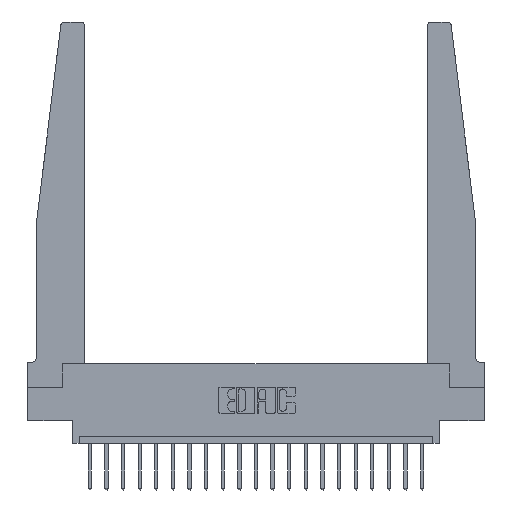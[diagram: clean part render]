
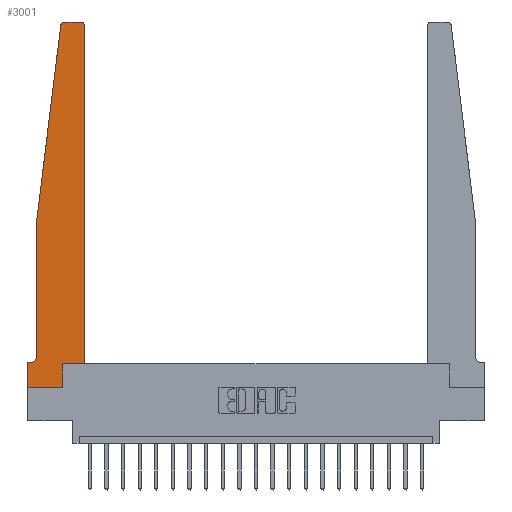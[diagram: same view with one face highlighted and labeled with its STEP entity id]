
A CAD part, top view. The second image highlights one B-rep face of the part: STEP entity #3001.
In plain terms, the highlighted planar face has unit normal (0, 0, 1).
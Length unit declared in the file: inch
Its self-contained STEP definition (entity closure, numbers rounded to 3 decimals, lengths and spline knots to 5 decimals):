
#333 = CARTESIAN_POINT ( 'NONE',  ( 0.015, 0.1875, 0.37 ) ) ;
#1010 = VECTOR ( 'NONE', #8053, 39.37008 ) ;
#1022 = PLANE ( 'NONE',  #12122 ) ;
#1224 = CARTESIAN_POINT ( 'NONE',  ( 0., 0.1875, 0.37 ) ) ;
#1341 = VERTEX_POINT ( 'NONE', #3713 ) ;
#1450 = VECTOR ( 'NONE', #2844, 39.37008 ) ;
#1490 = VERTEX_POINT ( 'NONE', #19080 ) ;
#1991 = CARTESIAN_POINT ( 'NONE',  ( 0.24675, 2.72367, 0.37 ) ) ;
#2009 = LINE ( 'NONE', #3826, #7385 ) ;
#2108 = ORIENTED_EDGE ( 'NONE', *, *, #13648, .T. ) ;
#2255 = CARTESIAN_POINT ( 'NONE',  ( 0.065, 0.2375, 0.37 ) ) ;
#2844 = DIRECTION ( 'NONE',  ( 0., -1., 0. ) ) ;
#3001 = ADVANCED_FACE ( 'NONE', ( #9588 ), #1022, .T. ) ;
#3008 = CARTESIAN_POINT ( 'NONE',  ( 0., 0.1875, 0.37 ) ) ;
#3049 = CARTESIAN_POINT ( 'NONE',  ( 0.065, 0.1875, 0.37 ) ) ;
#3063 = LINE ( 'NONE', #8006, #19202 ) ;
#3083 = ORIENTED_EDGE ( 'NONE', *, *, #13644, .T. ) ;
#3428 = CARTESIAN_POINT ( 'NONE',  ( 0.2605, 0.18, 0.37 ) ) ;
#3634 = ORIENTED_EDGE ( 'NONE', *, *, #11087, .T. ) ;
#3713 = CARTESIAN_POINT ( 'NONE',  ( 0.425, 2.72, 0.37 ) ) ;
#3826 = CARTESIAN_POINT ( 'NONE',  ( 0., 0., 0.37 ) ) ;
#4014 = VECTOR ( 'NONE', #17731, 39.37008 ) ;
#4241 = CARTESIAN_POINT ( 'NONE',  ( 0.27653, 2.75, 0.37 ) ) ;
#5000 = VECTOR ( 'NONE', #10655, 39.37008 ) ;
#5404 = CARTESIAN_POINT ( 'NONE',  ( 0., 0., 0.37 ) ) ;
#5937 = VERTEX_POINT ( 'NONE', #4241 ) ;
#5967 = DIRECTION ( 'NONE',  ( 0., 0., -1. ) ) ;
#6072 = CARTESIAN_POINT ( 'NONE',  ( 0., 0., 0.37 ) ) ;
#6158 = LINE ( 'NONE', #12679, #13641 ) ;
#6298 = VERTEX_POINT ( 'NONE', #3008 ) ;
#7385 = VECTOR ( 'NONE', #16719, 39.37008 ) ;
#7458 = AXIS2_PLACEMENT_3D ( 'NONE', #17946, #7973, #19352 ) ;
#7587 = VERTEX_POINT ( 'NONE', #2255 ) ;
#7666 = ORIENTED_EDGE ( 'NONE', *, *, #9296, .T. ) ;
#7973 = DIRECTION ( 'NONE',  ( 0., 0., 1. ) ) ;
#8006 = CARTESIAN_POINT ( 'NONE',  ( 0.065, 1.25, 0.37 ) ) ;
#8022 = ORIENTED_EDGE ( 'NONE', *, *, #17129, .T. ) ;
#8035 = CARTESIAN_POINT ( 'NONE',  ( 0.2605, 0., 0.37 ) ) ;
#8053 = DIRECTION ( 'NONE',  ( 0., 1., 0. ) ) ;
#8662 = EDGE_CURVE ( 'NONE', #17371, #16369, #2009, .T. ) ;
#9296 = EDGE_CURVE ( 'NONE', #13690, #5937, #17333, .T. ) ;
#9581 = DIRECTION ( 'NONE',  ( 1., 0., 0. ) ) ;
#9588 = FACE_OUTER_BOUND ( 'NONE', #10808, .T. ) ;
#9617 = CARTESIAN_POINT ( 'NONE',  ( 0.27653, 2.72, 0.37 ) ) ;
#9764 = ORIENTED_EDGE ( 'NONE', *, *, #12381, .T. ) ;
#10095 = VERTEX_POINT ( 'NONE', #15756 ) ;
#10655 = DIRECTION ( 'NONE',  ( -1., 0., 0. ) ) ;
#10656 = CARTESIAN_POINT ( 'NONE',  ( 0.015, 0.2375, 0.37 ) ) ;
#10808 = EDGE_LOOP ( 'NONE', ( #7666, #12319, #2108, #3634, #8022, #19317, #12587, #10823, #12771, #9764, #3083, #17591 ) ) ;
#10823 = ORIENTED_EDGE ( 'NONE', *, *, #8662, .T. ) ;
#11057 = EDGE_CURVE ( 'NONE', #1341, #13690, #15687, .T. ) ;
#11087 = EDGE_CURVE ( 'NONE', #18530, #7587, #14510, .T. ) ;
#11091 = CARTESIAN_POINT ( 'NONE',  ( 0.425, 0.18, 0.37 ) ) ;
#11159 = CARTESIAN_POINT ( 'NONE',  ( 0.065, 1.25, 0.37 ) ) ;
#11291 = VERTEX_POINT ( 'NONE', #333 ) ;
#11306 = LINE ( 'NONE', #11091, #15420 ) ;
#11911 = DIRECTION ( 'NONE',  ( 1., 0., 0. ) ) ;
#12122 = AXIS2_PLACEMENT_3D ( 'NONE', #1224, #15833, #17431 ) ;
#12319 = ORIENTED_EDGE ( 'NONE', *, *, #15755, .T. ) ;
#12381 = EDGE_CURVE ( 'NONE', #1490, #10095, #6158, .T. ) ;
#12587 = ORIENTED_EDGE ( 'NONE', *, *, #17140, .T. ) ;
#12679 = CARTESIAN_POINT ( 'NONE',  ( 0.425, 0.18, 0.37 ) ) ;
#12771 = ORIENTED_EDGE ( 'NONE', *, *, #12784, .T. ) ;
#12784 = EDGE_CURVE ( 'NONE', #16369, #1490, #19767, .T. ) ;
#13641 = VECTOR ( 'NONE', #9581, 39.37008 ) ;
#13644 = EDGE_CURVE ( 'NONE', #10095, #1341, #11306, .T. ) ;
#13648 = EDGE_CURVE ( 'NONE', #20662, #18530, #3063, .T. ) ;
#13690 = VERTEX_POINT ( 'NONE', #16057 ) ;
#14204 = DIRECTION ( 'NONE',  ( -1., 0., 0. ) ) ;
#14510 = LINE ( 'NONE', #11159, #4014 ) ;
#14543 = DIRECTION ( 'NONE',  ( -0.122, -0.992, 0. ) ) ;
#14750 = DIRECTION ( 'NONE',  ( 0., 1., 0. ) ) ;
#14859 = VECTOR ( 'NONE', #17550, 39.37008 ) ;
#15151 = DIRECTION ( 'NONE',  ( 0., 0., 1. ) ) ;
#15420 = VECTOR ( 'NONE', #14750, 39.37008 ) ;
#15502 = CIRCLE ( 'NONE', #18238, 0.05 ) ;
#15687 = CIRCLE ( 'NONE', #7458, 0.03 ) ;
#15755 = EDGE_CURVE ( 'NONE', #5937, #20662, #17175, .T. ) ;
#15756 = CARTESIAN_POINT ( 'NONE',  ( 0.425, 0.18, 0.37 ) ) ;
#15800 = AXIS2_PLACEMENT_3D ( 'NONE', #9617, #15151, #11911 ) ;
#15833 = DIRECTION ( 'NONE',  ( 0., 0., 1. ) ) ;
#16057 = CARTESIAN_POINT ( 'NONE',  ( 0.395, 2.75, 0.37 ) ) ;
#16156 = LINE ( 'NONE', #3049, #14859 ) ;
#16369 = VERTEX_POINT ( 'NONE', #8035 ) ;
#16719 = DIRECTION ( 'NONE',  ( 1., 0., 0. ) ) ;
#17129 = EDGE_CURVE ( 'NONE', #7587, #11291, #15502, .T. ) ;
#17140 = EDGE_CURVE ( 'NONE', #6298, #17371, #20773, .T. ) ;
#17175 = CIRCLE ( 'NONE', #15800, 0.03 ) ;
#17333 = LINE ( 'NONE', #18830, #5000 ) ;
#17371 = VERTEX_POINT ( 'NONE', #5404 ) ;
#17431 = DIRECTION ( 'NONE',  ( 1., 0., 0. ) ) ;
#17550 = DIRECTION ( 'NONE',  ( -1., 0., 0. ) ) ;
#17591 = ORIENTED_EDGE ( 'NONE', *, *, #11057, .T. ) ;
#17731 = DIRECTION ( 'NONE',  ( 0., -1., 0. ) ) ;
#17946 = CARTESIAN_POINT ( 'NONE',  ( 0.395, 2.72, 0.37 ) ) ;
#18238 = AXIS2_PLACEMENT_3D ( 'NONE', #10656, #5967, #14204 ) ;
#18530 = VERTEX_POINT ( 'NONE', #19807 ) ;
#18830 = CARTESIAN_POINT ( 'NONE',  ( 0.25, 2.75, 0.37 ) ) ;
#19080 = CARTESIAN_POINT ( 'NONE',  ( 0.2605, 0.18, 0.37 ) ) ;
#19202 = VECTOR ( 'NONE', #14543, 39.37008 ) ;
#19317 = ORIENTED_EDGE ( 'NONE', *, *, #20960, .T. ) ;
#19352 = DIRECTION ( 'NONE',  ( 1., 0., 0. ) ) ;
#19767 = LINE ( 'NONE', #3428, #1010 ) ;
#19807 = CARTESIAN_POINT ( 'NONE',  ( 0.065, 1.25, 0.37 ) ) ;
#20662 = VERTEX_POINT ( 'NONE', #1991 ) ;
#20773 = LINE ( 'NONE', #6072, #1450 ) ;
#20960 = EDGE_CURVE ( 'NONE', #11291, #6298, #16156, .T. ) ;
